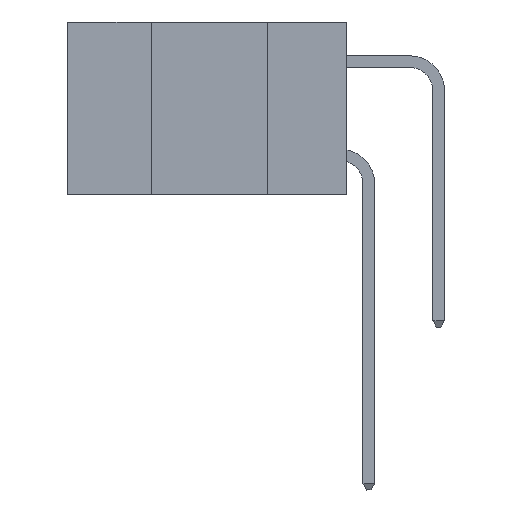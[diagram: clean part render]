
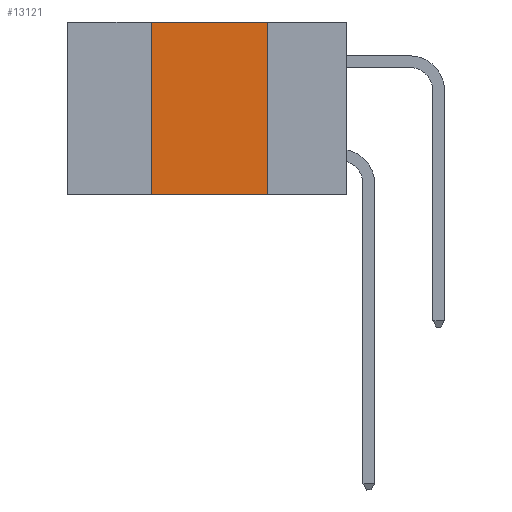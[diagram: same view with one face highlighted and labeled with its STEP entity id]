
A CAD part, left-side view. The second image highlights one B-rep face of the part: STEP entity #13121.
In plain terms, the highlighted planar face has unit normal (-1, 0, 0).
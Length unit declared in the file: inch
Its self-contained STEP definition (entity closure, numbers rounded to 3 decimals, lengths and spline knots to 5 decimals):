
#142 = CARTESIAN_POINT ( 'NONE',  ( 0., 0.17, 0. ) ) ;
#492 = DIRECTION ( 'NONE',  ( 0., 0., -1. ) ) ;
#2952 = LINE ( 'NONE', #4830, #8197 ) ;
#4247 = CARTESIAN_POINT ( 'NONE',  ( 0., 0.42, 0. ) ) ;
#4324 = ORIENTED_EDGE ( 'NONE', *, *, #17645, .F. ) ;
#4426 = VECTOR ( 'NONE', #20505, 39.37008 ) ;
#4830 = CARTESIAN_POINT ( 'NONE',  ( 0., 0.6, 0. ) ) ;
#5207 = CARTESIAN_POINT ( 'NONE',  ( 0., 0.17, -0.37 ) ) ;
#5744 = EDGE_CURVE ( 'NONE', #25227, #24791, #2952, .T. ) ;
#6721 = VECTOR ( 'NONE', #14060, 39.37008 ) ;
#7522 = FACE_OUTER_BOUND ( 'NONE', #15437, .T. ) ;
#7591 = EDGE_CURVE ( 'NONE', #24563, #13091, #14901, .T. ) ;
#8026 = EDGE_CURVE ( 'NONE', #24791, #13091, #16726, .T. ) ;
#8197 = VECTOR ( 'NONE', #22787, 39.37008 ) ;
#8699 = CARTESIAN_POINT ( 'NONE',  ( 0., 0.42, -0.37 ) ) ;
#9004 = VECTOR ( 'NONE', #492, 39.37008 ) ;
#10914 = PLANE ( 'NONE',  #18759 ) ;
#11249 = DIRECTION ( 'NONE',  ( 1., 0., 0. ) ) ;
#11977 = LINE ( 'NONE', #4247, #6721 ) ;
#13091 = VERTEX_POINT ( 'NONE', #5207 ) ;
#13121 = ADVANCED_FACE ( 'NONE', ( #7522 ), #10914, .F. ) ;
#14060 = DIRECTION ( 'NONE',  ( 0., 0., 1. ) ) ;
#14901 = LINE ( 'NONE', #16366, #4426 ) ;
#15004 = CARTESIAN_POINT ( 'NONE',  ( 0., 0.42, 0. ) ) ;
#15437 = EDGE_LOOP ( 'NONE', ( #22339, #16084, #4324, #16430 ) ) ;
#16084 = ORIENTED_EDGE ( 'NONE', *, *, #5744, .F. ) ;
#16366 = CARTESIAN_POINT ( 'NONE',  ( 0., 0.6, -0.37 ) ) ;
#16430 = ORIENTED_EDGE ( 'NONE', *, *, #7591, .T. ) ;
#16726 = LINE ( 'NONE', #142, #9004 ) ;
#17645 = EDGE_CURVE ( 'NONE', #24563, #25227, #11977, .T. ) ;
#18759 = AXIS2_PLACEMENT_3D ( 'NONE', #24746, #11249, #19320 ) ;
#19320 = DIRECTION ( 'NONE',  ( 0., 0., -1. ) ) ;
#20505 = DIRECTION ( 'NONE',  ( 0., -1., 0. ) ) ;
#21290 = CARTESIAN_POINT ( 'NONE',  ( 0., 0.17, 0. ) ) ;
#22339 = ORIENTED_EDGE ( 'NONE', *, *, #8026, .F. ) ;
#22787 = DIRECTION ( 'NONE',  ( 0., -1., 0. ) ) ;
#24563 = VERTEX_POINT ( 'NONE', #8699 ) ;
#24746 = CARTESIAN_POINT ( 'NONE',  ( 0., 0.6, 0. ) ) ;
#24791 = VERTEX_POINT ( 'NONE', #21290 ) ;
#25227 = VERTEX_POINT ( 'NONE', #15004 ) ;
